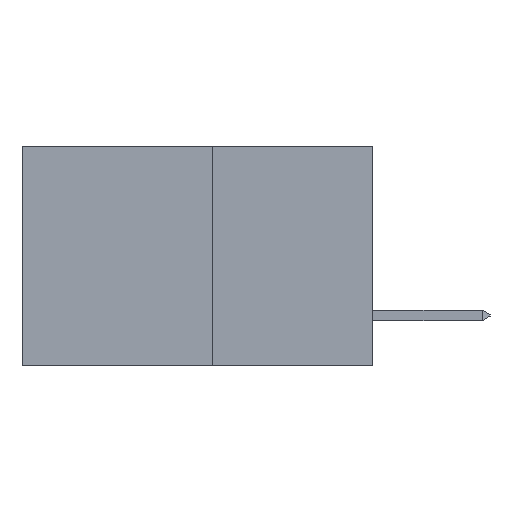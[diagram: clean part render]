
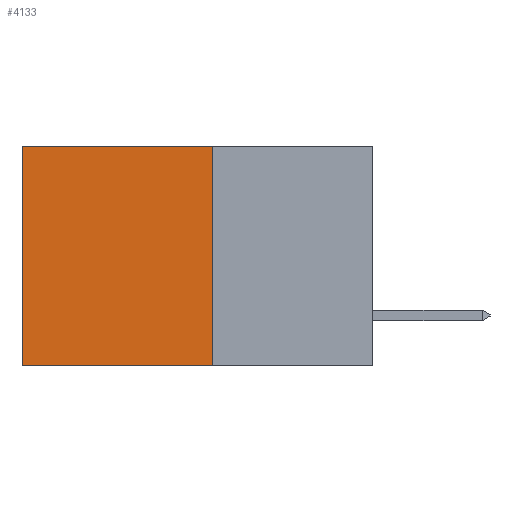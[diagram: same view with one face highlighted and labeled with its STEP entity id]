
A CAD part, left-side view. The second image highlights one B-rep face of the part: STEP entity #4133.
In plain terms, the highlighted planar face has unit normal (-1, 0, 0).
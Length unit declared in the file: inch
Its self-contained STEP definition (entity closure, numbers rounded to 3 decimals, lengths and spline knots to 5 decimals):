
#36 = CARTESIAN_POINT ( 'NONE',  ( 0.277, 0.27, -0.37 ) ) ;
#100 = ORIENTED_EDGE ( 'NONE', *, *, #2351, .T. ) ;
#233 = PLANE ( 'NONE',  #8166 ) ;
#361 = CARTESIAN_POINT ( 'NONE',  ( 0.277, 0.59, -0.37 ) ) ;
#734 = DIRECTION ( 'NONE',  ( 1., 0., 0. ) ) ;
#851 = CARTESIAN_POINT ( 'NONE',  ( 0.277, 0.27, -0.37 ) ) ;
#1192 = EDGE_LOOP ( 'NONE', ( #100, #2452, #5948, #6206 ) ) ;
#1772 = VERTEX_POINT ( 'NONE', #5225 ) ;
#2189 = DIRECTION ( 'NONE',  ( 0., 0., -1. ) ) ;
#2351 = EDGE_CURVE ( 'NONE', #5439, #9619, #3401, .T. ) ;
#2452 = ORIENTED_EDGE ( 'NONE', *, *, #3748, .F. ) ;
#2653 = FACE_OUTER_BOUND ( 'NONE', #1192, .T. ) ;
#3401 = LINE ( 'NONE', #4649, #7763 ) ;
#3554 = CARTESIAN_POINT ( 'NONE',  ( 0.277, 0.59, 0. ) ) ;
#3639 = DIRECTION ( 'NONE',  ( 0., 1., 0. ) ) ;
#3740 = VECTOR ( 'NONE', #6662, 39.37008 ) ;
#3748 = EDGE_CURVE ( 'NONE', #1772, #9619, #8924, .T. ) ;
#4133 = ADVANCED_FACE ( 'NONE', ( #2653 ), #233, .F. ) ;
#4597 = VECTOR ( 'NONE', #3639, 39.37008 ) ;
#4649 = CARTESIAN_POINT ( 'NONE',  ( 0.277, 0.59, -0.37 ) ) ;
#4703 = DIRECTION ( 'NONE',  ( 0., 0., -1. ) ) ;
#5225 = CARTESIAN_POINT ( 'NONE',  ( 0.277, 0.27, -0.37 ) ) ;
#5439 = VERTEX_POINT ( 'NONE', #3554 ) ;
#5948 = ORIENTED_EDGE ( 'NONE', *, *, #9924, .F. ) ;
#6206 = ORIENTED_EDGE ( 'NONE', *, *, #6931, .T. ) ;
#6627 = CARTESIAN_POINT ( 'NONE',  ( 0.277, 0.27, 0. ) ) ;
#6662 = DIRECTION ( 'NONE',  ( 0., 1., 0. ) ) ;
#6931 = EDGE_CURVE ( 'NONE', #10135, #5439, #10218, .T. ) ;
#7502 = DIRECTION ( 'NONE',  ( 0., 0., -1. ) ) ;
#7763 = VECTOR ( 'NONE', #4703, 39.37008 ) ;
#8166 = AXIS2_PLACEMENT_3D ( 'NONE', #36, #734, #2189 ) ;
#8840 = LINE ( 'NONE', #851, #10443 ) ;
#8924 = LINE ( 'NONE', #9641, #4597 ) ;
#9619 = VERTEX_POINT ( 'NONE', #361 ) ;
#9641 = CARTESIAN_POINT ( 'NONE',  ( 0.277, 0.27, -0.37 ) ) ;
#9924 = EDGE_CURVE ( 'NONE', #10135, #1772, #8840, .T. ) ;
#10118 = CARTESIAN_POINT ( 'NONE',  ( 0.277, 0.27, 0. ) ) ;
#10135 = VERTEX_POINT ( 'NONE', #10118 ) ;
#10218 = LINE ( 'NONE', #6627, #3740 ) ;
#10443 = VECTOR ( 'NONE', #7502, 39.37008 ) ;
